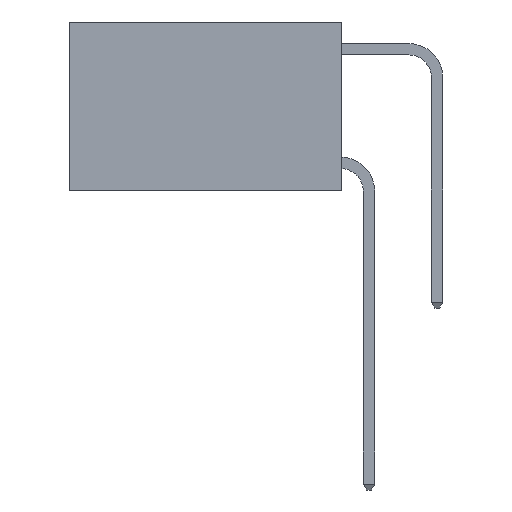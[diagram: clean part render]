
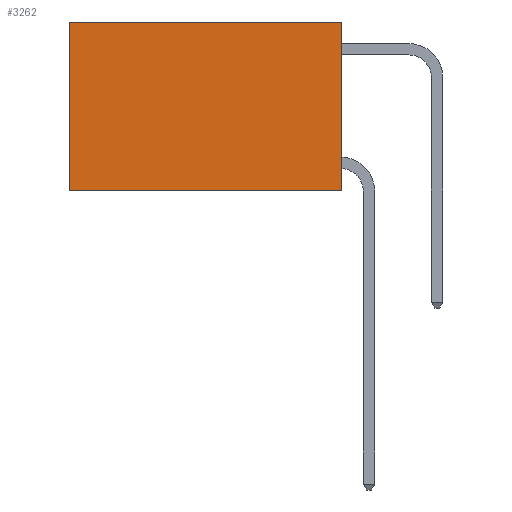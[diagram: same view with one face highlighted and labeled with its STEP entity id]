
A CAD part, left-side view. The second image highlights one B-rep face of the part: STEP entity #3262.
In plain terms, the highlighted planar face has unit normal (-1, 0, 0).
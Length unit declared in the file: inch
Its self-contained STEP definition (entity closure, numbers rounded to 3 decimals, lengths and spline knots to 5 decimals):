
#391 = AXIS2_PLACEMENT_3D ( 'NONE', #4107, #10503, #5036 ) ;
#1071 = ORIENTED_EDGE ( 'NONE', *, *, #7593, .F. ) ;
#1155 = CARTESIAN_POINT ( 'NONE',  ( 0.2625, 0., -0.37 ) ) ;
#1254 = CARTESIAN_POINT ( 'NONE',  ( 0.2625, 0., 0. ) ) ;
#1926 = DIRECTION ( 'NONE',  ( 0., 0., -1. ) ) ;
#2062 = EDGE_CURVE ( 'NONE', #11113, #9059, #4897, .T. ) ;
#2731 = ORIENTED_EDGE ( 'NONE', *, *, #2062, .F. ) ;
#3164 = LINE ( 'NONE', #3658, #8363 ) ;
#3262 = ADVANCED_FACE ( 'NONE', ( #5725 ), #11384, .F. ) ;
#3405 = CARTESIAN_POINT ( 'NONE',  ( 0.2625, 0.6, 0. ) ) ;
#3658 = CARTESIAN_POINT ( 'NONE',  ( 0.2625, 0., 0. ) ) ;
#4107 = CARTESIAN_POINT ( 'NONE',  ( 0.2625, 0., 0. ) ) ;
#4897 = LINE ( 'NONE', #1155, #8894 ) ;
#5036 = DIRECTION ( 'NONE',  ( 0., 0., -1. ) ) ;
#5690 = CARTESIAN_POINT ( 'NONE',  ( 0.2625, 0., 0. ) ) ;
#5725 = FACE_OUTER_BOUND ( 'NONE', #9627, .T. ) ;
#6291 = EDGE_CURVE ( 'NONE', #8571, #9059, #8840, .T. ) ;
#6662 = LINE ( 'NONE', #5690, #11517 ) ;
#6781 = DIRECTION ( 'NONE',  ( 0., 1., 0. ) ) ;
#7453 = EDGE_CURVE ( 'NONE', #10983, #8571, #3164, .T. ) ;
#7593 = EDGE_CURVE ( 'NONE', #10983, #11113, #6662, .T. ) ;
#8363 = VECTOR ( 'NONE', #10076, 39.37008 ) ;
#8571 = VERTEX_POINT ( 'NONE', #3405 ) ;
#8668 = CARTESIAN_POINT ( 'NONE',  ( 0.2625, 0.6, 0. ) ) ;
#8840 = LINE ( 'NONE', #8668, #10973 ) ;
#8894 = VECTOR ( 'NONE', #6781, 39.37008 ) ;
#8909 = CARTESIAN_POINT ( 'NONE',  ( 0.2625, 0., -0.37 ) ) ;
#9059 = VERTEX_POINT ( 'NONE', #11402 ) ;
#9317 = ORIENTED_EDGE ( 'NONE', *, *, #6291, .T. ) ;
#9627 = EDGE_LOOP ( 'NONE', ( #9317, #2731, #1071, #11651 ) ) ;
#10076 = DIRECTION ( 'NONE',  ( 0., 1., 0. ) ) ;
#10503 = DIRECTION ( 'NONE',  ( 1., 0., 0. ) ) ;
#10973 = VECTOR ( 'NONE', #11426, 39.37008 ) ;
#10983 = VERTEX_POINT ( 'NONE', #1254 ) ;
#11113 = VERTEX_POINT ( 'NONE', #8909 ) ;
#11384 = PLANE ( 'NONE',  #391 ) ;
#11402 = CARTESIAN_POINT ( 'NONE',  ( 0.2625, 0.6, -0.37 ) ) ;
#11426 = DIRECTION ( 'NONE',  ( 0., 0., -1. ) ) ;
#11517 = VECTOR ( 'NONE', #1926, 39.37008 ) ;
#11651 = ORIENTED_EDGE ( 'NONE', *, *, #7453, .T. ) ;
